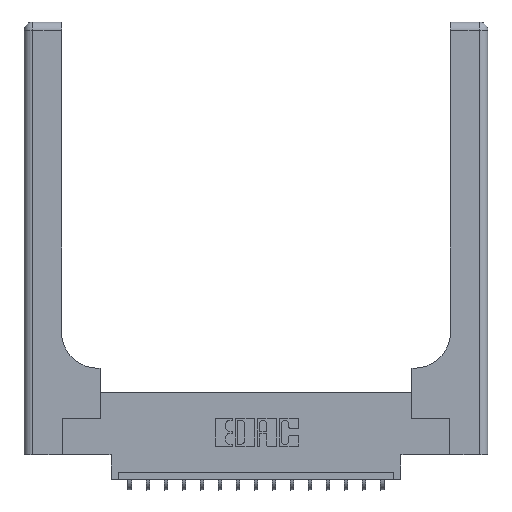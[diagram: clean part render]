
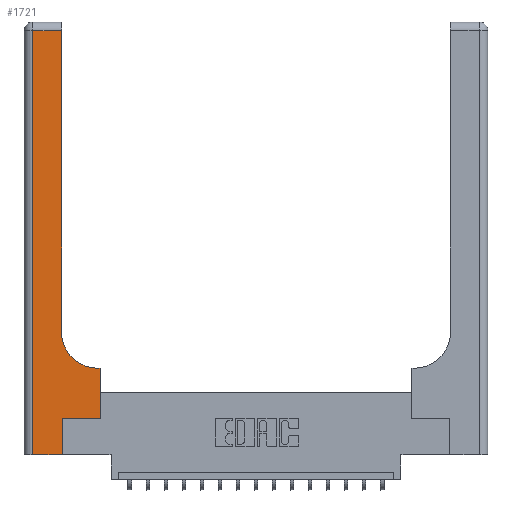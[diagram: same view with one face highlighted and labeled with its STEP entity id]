
A CAD part, top view. The second image highlights one B-rep face of the part: STEP entity #1721.
In plain terms, the highlighted planar face has unit normal (0, 0, 1).
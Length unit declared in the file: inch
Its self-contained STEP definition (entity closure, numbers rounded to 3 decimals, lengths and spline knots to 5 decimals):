
#593 = VECTOR ( 'NONE', #1321, 39.37008 ) ;
#701 = DIRECTION ( 'NONE',  ( 1., 0., 0. ) ) ;
#860 = CARTESIAN_POINT ( 'NONE',  ( 0.528, 0.6, 0.37 ) ) ;
#941 = DIRECTION ( 'NONE',  ( 0., -1., 0. ) ) ;
#1134 = LINE ( 'NONE', #14355, #593 ) ;
#1241 = ORIENTED_EDGE ( 'NONE', *, *, #4533, .T. ) ;
#1321 = DIRECTION ( 'NONE',  ( 1., 0., 0. ) ) ;
#1352 = CARTESIAN_POINT ( 'NONE',  ( 0.265, 0., 0.37 ) ) ;
#1577 = CARTESIAN_POINT ( 'NONE',  ( 0.26, 0.85, 0.37 ) ) ;
#1721 = ADVANCED_FACE ( 'NONE', ( #9043 ), #13415, .F. ) ;
#1846 = CARTESIAN_POINT ( 'NONE',  ( 0.265, 0.25, 0.37 ) ) ;
#1944 = CARTESIAN_POINT ( 'NONE',  ( 0.265, 0., 0.37 ) ) ;
#2038 = CARTESIAN_POINT ( 'NONE',  ( 0.51, 0.6, 0.37 ) ) ;
#2603 = CARTESIAN_POINT ( 'NONE',  ( 0.06, 2.94, 0.37 ) ) ;
#2636 = AXIS2_PLACEMENT_3D ( 'NONE', #3332, #10369, #16184 ) ;
#3332 = CARTESIAN_POINT ( 'NONE',  ( 0., 3., 0.37 ) ) ;
#3458 = LINE ( 'NONE', #1944, #18615 ) ;
#3642 = EDGE_CURVE ( 'NONE', #11647, #8648, #12817, .T. ) ;
#3645 = LINE ( 'NONE', #14020, #11784 ) ;
#3762 = ORIENTED_EDGE ( 'NONE', *, *, #6343, .T. ) ;
#4006 = VERTEX_POINT ( 'NONE', #1352 ) ;
#4224 = LINE ( 'NONE', #7071, #6939 ) ;
#4241 = ORIENTED_EDGE ( 'NONE', *, *, #18221, .T. ) ;
#4533 = EDGE_CURVE ( 'NONE', #18079, #13249, #16354, .T. ) ;
#5398 = CARTESIAN_POINT ( 'NONE',  ( 0.528, 0.25, 0.37 ) ) ;
#5848 = AXIS2_PLACEMENT_3D ( 'NONE', #13365, #7637, #12221 ) ;
#6063 = VERTEX_POINT ( 'NONE', #14126 ) ;
#6321 = EDGE_CURVE ( 'NONE', #13249, #8739, #6458, .T. ) ;
#6343 = EDGE_CURVE ( 'NONE', #4006, #8703, #3458, .T. ) ;
#6458 = CIRCLE ( 'NONE', #5848, 0.25 ) ;
#6648 = VECTOR ( 'NONE', #941, 39.37008 ) ;
#6939 = VECTOR ( 'NONE', #17542, 39.37008 ) ;
#6964 = EDGE_CURVE ( 'NONE', #8648, #6063, #9665, .T. ) ;
#7071 = CARTESIAN_POINT ( 'NONE',  ( 0.26, 3., 0.37 ) ) ;
#7478 = EDGE_CURVE ( 'NONE', #8739, #11647, #4224, .T. ) ;
#7637 = DIRECTION ( 'NONE',  ( 0., 0., -1. ) ) ;
#8206 = VECTOR ( 'NONE', #14339, 39.37008 ) ;
#8529 = CARTESIAN_POINT ( 'NONE',  ( 0.06, 3., 0.37 ) ) ;
#8648 = VERTEX_POINT ( 'NONE', #2603 ) ;
#8703 = VERTEX_POINT ( 'NONE', #18396 ) ;
#8739 = VERTEX_POINT ( 'NONE', #1577 ) ;
#9043 = FACE_OUTER_BOUND ( 'NONE', #14628, .T. ) ;
#9199 = VECTOR ( 'NONE', #12166, 39.37008 ) ;
#9665 = LINE ( 'NONE', #8529, #6648 ) ;
#10042 = ORIENTED_EDGE ( 'NONE', *, *, #6321, .T. ) ;
#10369 = DIRECTION ( 'NONE',  ( 0., 0., -1. ) ) ;
#10916 = VERTEX_POINT ( 'NONE', #5398 ) ;
#11647 = VERTEX_POINT ( 'NONE', #11858 ) ;
#11784 = VECTOR ( 'NONE', #18103, 39.37008 ) ;
#11858 = CARTESIAN_POINT ( 'NONE',  ( 0.26, 2.94, 0.37 ) ) ;
#12166 = DIRECTION ( 'NONE',  ( -1., 0., 0. ) ) ;
#12221 = DIRECTION ( 'NONE',  ( 1., 0., 0. ) ) ;
#12817 = LINE ( 'NONE', #14239, #8206 ) ;
#12956 = ORIENTED_EDGE ( 'NONE', *, *, #14543, .T. ) ;
#13197 = ORIENTED_EDGE ( 'NONE', *, *, #3642, .T. ) ;
#13249 = VERTEX_POINT ( 'NONE', #2038 ) ;
#13365 = CARTESIAN_POINT ( 'NONE',  ( 0.51, 0.85, 0.37 ) ) ;
#13415 = PLANE ( 'NONE',  #2636 ) ;
#13586 = CARTESIAN_POINT ( 'NONE',  ( 0.26, 0.6, 0.37 ) ) ;
#14020 = CARTESIAN_POINT ( 'NONE',  ( 0.528, 0.25, 0.37 ) ) ;
#14126 = CARTESIAN_POINT ( 'NONE',  ( 0.06, 0., 0.37 ) ) ;
#14239 = CARTESIAN_POINT ( 'NONE',  ( 0., 2.94, 0.37 ) ) ;
#14339 = DIRECTION ( 'NONE',  ( -1., 0., 0. ) ) ;
#14355 = CARTESIAN_POINT ( 'NONE',  ( 0., 0., 0.37 ) ) ;
#14543 = EDGE_CURVE ( 'NONE', #10916, #18079, #3645, .T. ) ;
#14628 = EDGE_LOOP ( 'NONE', ( #17368, #13197, #16838, #4241, #3762, #17882, #12956, #1241, #10042 ) ) ;
#16184 = DIRECTION ( 'NONE',  ( -1., 0., 0. ) ) ;
#16217 = DIRECTION ( 'NONE',  ( 0., 1., 0. ) ) ;
#16306 = LINE ( 'NONE', #1846, #16392 ) ;
#16354 = LINE ( 'NONE', #13586, #9199 ) ;
#16392 = VECTOR ( 'NONE', #701, 39.37008 ) ;
#16838 = ORIENTED_EDGE ( 'NONE', *, *, #6964, .T. ) ;
#17368 = ORIENTED_EDGE ( 'NONE', *, *, #7478, .T. ) ;
#17542 = DIRECTION ( 'NONE',  ( 0., 1., 0. ) ) ;
#17882 = ORIENTED_EDGE ( 'NONE', *, *, #18642, .T. ) ;
#18079 = VERTEX_POINT ( 'NONE', #860 ) ;
#18103 = DIRECTION ( 'NONE',  ( 0., 1., 0. ) ) ;
#18221 = EDGE_CURVE ( 'NONE', #6063, #4006, #1134, .T. ) ;
#18396 = CARTESIAN_POINT ( 'NONE',  ( 0.265, 0.25, 0.37 ) ) ;
#18615 = VECTOR ( 'NONE', #16217, 39.37008 ) ;
#18642 = EDGE_CURVE ( 'NONE', #8703, #10916, #16306, .T. ) ;
